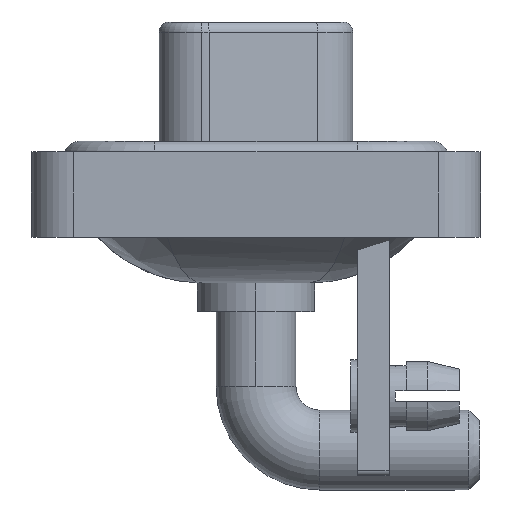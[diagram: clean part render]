
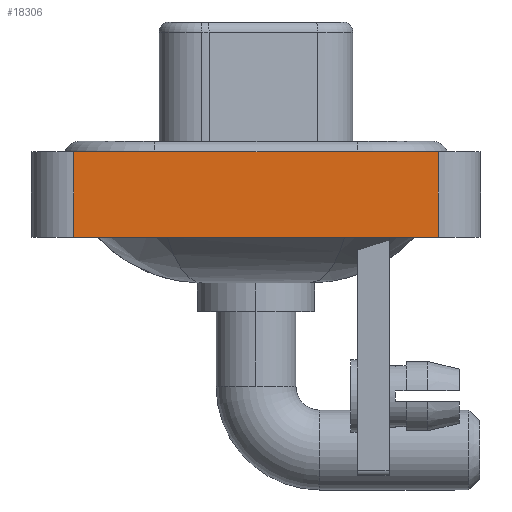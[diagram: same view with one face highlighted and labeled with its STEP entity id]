
A CAD part, left-side view. The second image highlights one B-rep face of the part: STEP entity #18306.
In plain terms, the highlighted planar face has unit normal (-1, 0, 0).
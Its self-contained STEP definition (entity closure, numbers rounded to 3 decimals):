
#503 = LINE ( 'NONE', #14767, #18442 ) ;
#528 = VECTOR ( 'NONE', #14425, 1000. ) ;
#1745 = VECTOR ( 'NONE', #18132, 1000. ) ;
#1799 = CARTESIAN_POINT ( 'NONE',  ( -7.25, 8.55, -3.6 ) ) ;
#3814 = DIRECTION ( 'NONE',  ( 0., 0., 1. ) ) ;
#4618 = DIRECTION ( 'NONE',  ( 0., 0., 1. ) ) ;
#5002 = VECTOR ( 'NONE', #13656, 1000. ) ;
#5971 = VERTEX_POINT ( 'NONE', #8684 ) ;
#6046 = FACE_OUTER_BOUND ( 'NONE', #15592, .T. ) ;
#6281 = VERTEX_POINT ( 'NONE', #1799 ) ;
#6649 = EDGE_CURVE ( 'NONE', #17420, #19958, #503, .T. ) ;
#6727 = CARTESIAN_POINT ( 'NONE',  ( -7.25, -8.55, -3.6 ) ) ;
#8057 = ORIENTED_EDGE ( 'NONE', *, *, #10660, .F. ) ;
#8684 = CARTESIAN_POINT ( 'NONE',  ( -7.25, 8.55, 0.4 ) ) ;
#8993 = CARTESIAN_POINT ( 'NONE',  ( -7.25, -8.55, -3.6 ) ) ;
#9319 = CARTESIAN_POINT ( 'NONE',  ( -7.25, -8.55, -3.6 ) ) ;
#10600 = AXIS2_PLACEMENT_3D ( 'NONE', #9319, #13748, #4618 ) ;
#10660 = EDGE_CURVE ( 'NONE', #6281, #5971, #15591, .T. ) ;
#10927 = EDGE_CURVE ( 'NONE', #5971, #19958, #17717, .T. ) ;
#11612 = ORIENTED_EDGE ( 'NONE', *, *, #20229, .T. ) ;
#12131 = ORIENTED_EDGE ( 'NONE', *, *, #6649, .T. ) ;
#13656 = DIRECTION ( 'NONE',  ( 0., 0., 1. ) ) ;
#13748 = DIRECTION ( 'NONE',  ( -1., 0., 0. ) ) ;
#14425 = DIRECTION ( 'NONE',  ( 0., -1., 0. ) ) ;
#14461 = ORIENTED_EDGE ( 'NONE', *, *, #10927, .F. ) ;
#14650 = CARTESIAN_POINT ( 'NONE',  ( -7.25, -8.55, 0.4 ) ) ;
#14767 = CARTESIAN_POINT ( 'NONE',  ( -7.25, -8.55, -3.6 ) ) ;
#15591 = LINE ( 'NONE', #17117, #5002 ) ;
#15592 = EDGE_LOOP ( 'NONE', ( #12131, #14461, #8057, #11612 ) ) ;
#15968 = LINE ( 'NONE', #6727, #528 ) ;
#17017 = PLANE ( 'NONE',  #10600 ) ;
#17117 = CARTESIAN_POINT ( 'NONE',  ( -7.25, 8.55, -3.6 ) ) ;
#17420 = VERTEX_POINT ( 'NONE', #8993 ) ;
#17717 = LINE ( 'NONE', #14650, #1745 ) ;
#18132 = DIRECTION ( 'NONE',  ( 0., -1., 0. ) ) ;
#18306 = ADVANCED_FACE ( 'NONE', ( #6046 ), #17017, .T. ) ;
#18442 = VECTOR ( 'NONE', #3814, 1000. ) ;
#19190 = CARTESIAN_POINT ( 'NONE',  ( -7.25, -8.55, 0.4 ) ) ;
#19958 = VERTEX_POINT ( 'NONE', #19190 ) ;
#20229 = EDGE_CURVE ( 'NONE', #6281, #17420, #15968, .T. ) ;
